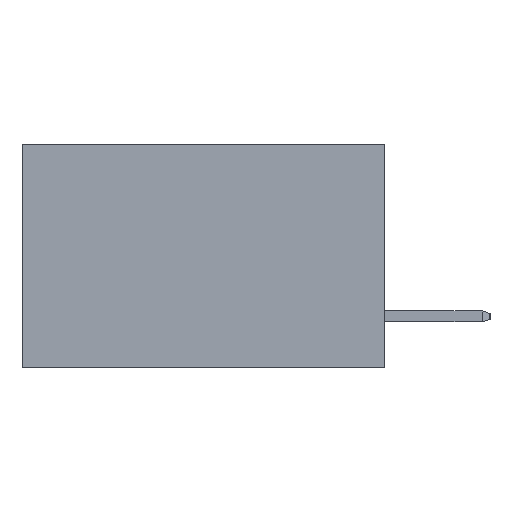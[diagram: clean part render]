
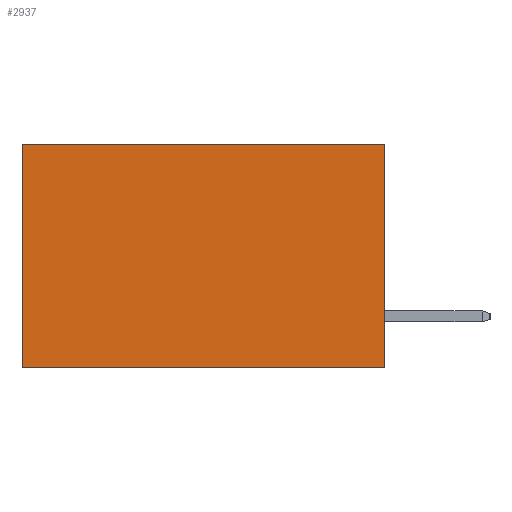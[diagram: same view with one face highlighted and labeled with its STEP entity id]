
A CAD part, left-side view. The second image highlights one B-rep face of the part: STEP entity #2937.
In plain terms, the highlighted planar face has unit normal (-1, 0, 0).
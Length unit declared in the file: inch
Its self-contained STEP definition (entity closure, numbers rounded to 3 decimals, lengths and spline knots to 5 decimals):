
#374 = ORIENTED_EDGE ( 'NONE', *, *, #4933, .T. ) ;
#424 = FACE_OUTER_BOUND ( 'NONE', #12791, .T. ) ;
#676 = CARTESIAN_POINT ( 'NONE',  ( 0.298, 0.6, -0.37 ) ) ;
#992 = VECTOR ( 'NONE', #14096, 39.37008 ) ;
#1018 = DIRECTION ( 'NONE',  ( 0., 1., 0. ) ) ;
#1359 = LINE ( 'NONE', #13030, #992 ) ;
#1371 = DIRECTION ( 'NONE',  ( 0., 1., 0. ) ) ;
#1780 = CARTESIAN_POINT ( 'NONE',  ( 0.298, 0., 0. ) ) ;
#1835 = DIRECTION ( 'NONE',  ( 0., 0., -1. ) ) ;
#1952 = CARTESIAN_POINT ( 'NONE',  ( 0.298, 0., -0.37 ) ) ;
#2523 = LINE ( 'NONE', #11142, #5190 ) ;
#2937 = ADVANCED_FACE ( 'NONE', ( #424 ), #9213, .F. ) ;
#3615 = CARTESIAN_POINT ( 'NONE',  ( 0.298, 0., -0.37 ) ) ;
#3857 = DIRECTION ( 'NONE',  ( 1., 0., 0. ) ) ;
#4933 = EDGE_CURVE ( 'NONE', #6262, #10437, #2523, .T. ) ;
#5190 = VECTOR ( 'NONE', #5311, 39.37008 ) ;
#5311 = DIRECTION ( 'NONE',  ( 0., 0., -1. ) ) ;
#5796 = CARTESIAN_POINT ( 'NONE',  ( 0.298, 0., 0. ) ) ;
#5819 = ORIENTED_EDGE ( 'NONE', *, *, #10470, .F. ) ;
#5976 = ORIENTED_EDGE ( 'NONE', *, *, #9285, .T. ) ;
#6262 = VERTEX_POINT ( 'NONE', #13473 ) ;
#6642 = AXIS2_PLACEMENT_3D ( 'NONE', #1780, #3857, #1835 ) ;
#9213 = PLANE ( 'NONE',  #6642 ) ;
#9285 = EDGE_CURVE ( 'NONE', #9449, #6262, #14386, .T. ) ;
#9449 = VERTEX_POINT ( 'NONE', #5796 ) ;
#9486 = VECTOR ( 'NONE', #1371, 39.37008 ) ;
#10437 = VERTEX_POINT ( 'NONE', #676 ) ;
#10470 = EDGE_CURVE ( 'NONE', #9449, #14116, #1359, .T. ) ;
#11142 = CARTESIAN_POINT ( 'NONE',  ( 0.298, 0.6, 0. ) ) ;
#11332 = EDGE_CURVE ( 'NONE', #14116, #10437, #12373, .T. ) ;
#11569 = VECTOR ( 'NONE', #1018, 39.37008 ) ;
#12197 = CARTESIAN_POINT ( 'NONE',  ( 0.298, 0., 0. ) ) ;
#12373 = LINE ( 'NONE', #3615, #9486 ) ;
#12791 = EDGE_LOOP ( 'NONE', ( #374, #13589, #5819, #5976 ) ) ;
#13030 = CARTESIAN_POINT ( 'NONE',  ( 0.298, 0., 0. ) ) ;
#13473 = CARTESIAN_POINT ( 'NONE',  ( 0.298, 0.6, 0. ) ) ;
#13589 = ORIENTED_EDGE ( 'NONE', *, *, #11332, .F. ) ;
#14096 = DIRECTION ( 'NONE',  ( 0., 0., -1. ) ) ;
#14116 = VERTEX_POINT ( 'NONE', #1952 ) ;
#14386 = LINE ( 'NONE', #12197, #11569 ) ;
